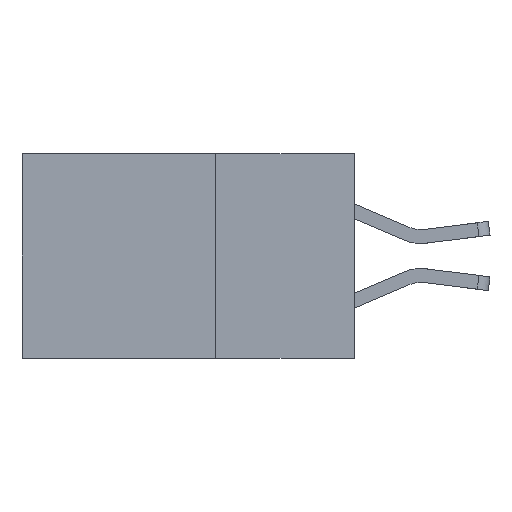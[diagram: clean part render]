
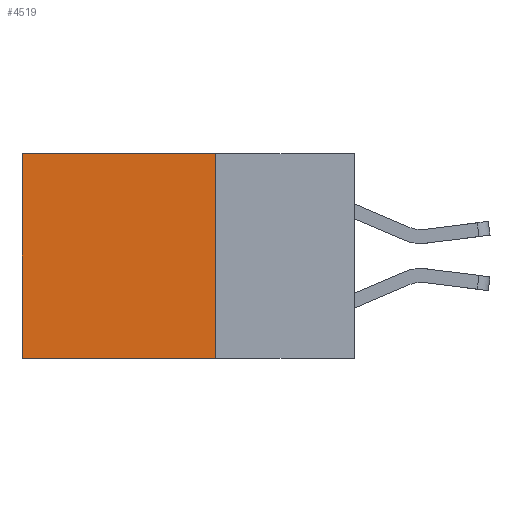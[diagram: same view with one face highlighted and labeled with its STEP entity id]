
A CAD part, left-side view. The second image highlights one B-rep face of the part: STEP entity #4519.
In plain terms, the highlighted planar face has unit normal (-1, 0, 0).
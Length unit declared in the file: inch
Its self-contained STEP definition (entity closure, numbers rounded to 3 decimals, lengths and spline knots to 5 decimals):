
#154 = VECTOR ( 'NONE', #8808, 39.37008 ) ;
#564 = AXIS2_PLACEMENT_3D ( 'NONE', #8212, #8150, #8143 ) ;
#1127 = CARTESIAN_POINT ( 'NONE',  ( 0.298, 0.25, -0.37 ) ) ;
#1848 = EDGE_LOOP ( 'NONE', ( #8739, #2516, #4656, #8997 ) ) ;
#2223 = LINE ( 'NONE', #9599, #154 ) ;
#2465 = LINE ( 'NONE', #3909, #8679 ) ;
#2516 = ORIENTED_EDGE ( 'NONE', *, *, #3615, .F. ) ;
#2523 = CARTESIAN_POINT ( 'NONE',  ( 0.298, 0.25, 0. ) ) ;
#2760 = DIRECTION ( 'NONE',  ( 0., 1., 0. ) ) ;
#3615 = EDGE_CURVE ( 'NONE', #8963, #7282, #10132, .T. ) ;
#3909 = CARTESIAN_POINT ( 'NONE',  ( 0.298, 0.25, 0. ) ) ;
#4015 = FACE_OUTER_BOUND ( 'NONE', #1848, .T. ) ;
#4090 = VECTOR ( 'NONE', #7277, 39.37008 ) ;
#4411 = VERTEX_POINT ( 'NONE', #8497 ) ;
#4519 = ADVANCED_FACE ( 'NONE', ( #4015 ), #8227, .F. ) ;
#4656 = ORIENTED_EDGE ( 'NONE', *, *, #8789, .F. ) ;
#5573 = CARTESIAN_POINT ( 'NONE',  ( 0.298, 0.25, 0. ) ) ;
#5896 = VECTOR ( 'NONE', #2760, 39.37008 ) ;
#6320 = LINE ( 'NONE', #5573, #4090 ) ;
#6511 = VERTEX_POINT ( 'NONE', #2523 ) ;
#6656 = CARTESIAN_POINT ( 'NONE',  ( 0.298, 0.25, -0.37 ) ) ;
#7277 = DIRECTION ( 'NONE',  ( 0., 0., -1. ) ) ;
#7282 = VERTEX_POINT ( 'NONE', #9873 ) ;
#7994 = DIRECTION ( 'NONE',  ( 0., 1., 0. ) ) ;
#8143 = DIRECTION ( 'NONE',  ( 0., 0., -1. ) ) ;
#8150 = DIRECTION ( 'NONE',  ( 1., 0., 0. ) ) ;
#8212 = CARTESIAN_POINT ( 'NONE',  ( 0.298, 0.25, 0. ) ) ;
#8227 = PLANE ( 'NONE',  #564 ) ;
#8497 = CARTESIAN_POINT ( 'NONE',  ( 0.298, 0.6, 0. ) ) ;
#8679 = VECTOR ( 'NONE', #7994, 39.37008 ) ;
#8739 = ORIENTED_EDGE ( 'NONE', *, *, #8776, .T. ) ;
#8741 = EDGE_CURVE ( 'NONE', #6511, #4411, #2465, .T. ) ;
#8776 = EDGE_CURVE ( 'NONE', #4411, #7282, #2223, .T. ) ;
#8789 = EDGE_CURVE ( 'NONE', #6511, #8963, #6320, .T. ) ;
#8808 = DIRECTION ( 'NONE',  ( 0., 0., -1. ) ) ;
#8963 = VERTEX_POINT ( 'NONE', #6656 ) ;
#8997 = ORIENTED_EDGE ( 'NONE', *, *, #8741, .T. ) ;
#9599 = CARTESIAN_POINT ( 'NONE',  ( 0.298, 0.6, 0. ) ) ;
#9873 = CARTESIAN_POINT ( 'NONE',  ( 0.298, 0.6, -0.37 ) ) ;
#10132 = LINE ( 'NONE', #1127, #5896 ) ;
